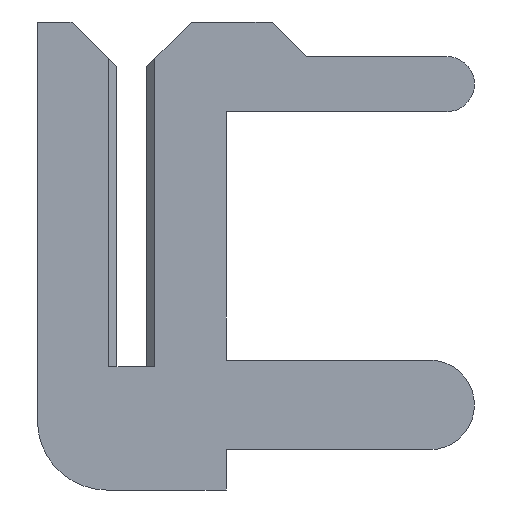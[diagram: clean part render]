
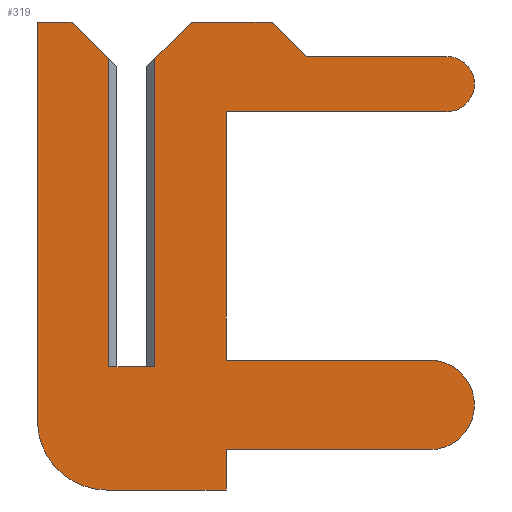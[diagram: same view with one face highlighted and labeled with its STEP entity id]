
A CAD part, left-side view. The second image highlights one B-rep face of the part: STEP entity #319.
In plain terms, the highlighted planar face has unit normal (-1, 0, 0).
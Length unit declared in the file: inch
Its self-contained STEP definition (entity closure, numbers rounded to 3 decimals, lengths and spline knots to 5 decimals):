
#2 = EDGE_CURVE ( 'NONE', #1011, #644, #802, .T. ) ;
#6 = AXIS2_PLACEMENT_3D ( 'NONE', #344, #510, #598 ) ;
#14 = LINE ( 'NONE', #711, #265 ) ;
#28 = EDGE_CURVE ( 'NONE', #370, #630, #1058, .T. ) ;
#31 = CIRCLE ( 'NONE', #512, 0.0195 ) ;
#42 = DIRECTION ( 'NONE',  ( 0., -1., 0. ) ) ;
#43 = EDGE_CURVE ( 'NONE', #541, #501, #550, .T. ) ;
#44 = CIRCLE ( 'NONE', #608, 0.03 ) ;
#46 = CARTESIAN_POINT ( 'NONE',  ( -0.01, -0.0065, 0.1305 ) ) ;
#52 = CARTESIAN_POINT ( 'NONE',  ( -0.01, 0.01, -0.0235 ) ) ;
#53 = CARTESIAN_POINT ( 'NONE',  ( -0.01, -0.1295, -0.0165 ) ) ;
#59 = EDGE_CURVE ( 'NONE', #644, #306, #841, .T. ) ;
#63 = PLANE ( 'NONE',  #1045 ) ;
#70 = CARTESIAN_POINT ( 'NONE',  ( -0.01, 0.011, -0.0235 ) ) ;
#73 = CARTESIAN_POINT ( 'NONE',  ( -0.01, -0.041, -0.036 ) ) ;
#79 = VERTEX_POINT ( 'NONE', #434 ) ;
#94 = CARTESIAN_POINT ( 'NONE',  ( -0.01, -0.137, 0.111 ) ) ;
#103 = LINE ( 'NONE', #46, #860 ) ;
#114 = CARTESIAN_POINT ( 'NONE',  ( -0.01, 0.041, 0.15 ) ) ;
#121 = ORIENTED_EDGE ( 'NONE', *, *, #570, .F. ) ;
#141 = DIRECTION ( 'NONE',  ( 0., 1., 0. ) ) ;
#142 = LINE ( 'NONE', #276, #324 ) ;
#153 = EDGE_CURVE ( 'NONE', #421, #204, #31, .T. ) ;
#160 = VECTOR ( 'NONE', #927, 39.37008 ) ;
#168 = EDGE_CURVE ( 'NONE', #865, #421, #820, .T. ) ;
#169 = LINE ( 'NONE', #288, #903 ) ;
#170 = EDGE_CURVE ( 'NONE', #611, #1011, #103, .T. ) ;
#179 = CARTESIAN_POINT ( 'NONE',  ( -0.01, 0.041, -0.0235 ) ) ;
#183 = LINE ( 'NONE', #674, #354 ) ;
#184 = LINE ( 'NONE', #73, #892 ) ;
#193 = DIRECTION ( 'NONE',  ( 0., 0., -1. ) ) ;
#204 = VERTEX_POINT ( 'NONE', #362 ) ;
#208 = DIRECTION ( 'NONE',  ( 0., 1., 0. ) ) ;
#217 = VECTOR ( 'NONE', #516, 39.37008 ) ;
#220 = ORIENTED_EDGE ( 'NONE', *, *, #698, .F. ) ;
#224 = CARTESIAN_POINT ( 'NONE',  ( -0.01, -0.01, 0. ) ) ;
#225 = DIRECTION ( 'NONE',  ( 0., 1., 0. ) ) ;
#247 = VERTEX_POINT ( 'NONE', #224 ) ;
#251 = EDGE_CURVE ( 'NONE', #501, #79, #14, .T. ) ;
#260 = ORIENTED_EDGE ( 'NONE', *, *, #59, .F. ) ;
#265 = VECTOR ( 'NONE', #525, 39.37008 ) ;
#273 = ORIENTED_EDGE ( 'NONE', *, *, #348, .F. ) ;
#276 = CARTESIAN_POINT ( 'NONE',  ( -0.01, -0.137, 0.135 ) ) ;
#277 = CARTESIAN_POINT ( 'NONE',  ( -0.01, -0.076, 0.135 ) ) ;
#282 = FACE_OUTER_BOUND ( 'NONE', #766, .T. ) ;
#288 = CARTESIAN_POINT ( 'NONE',  ( -0.01, -0.041, 0.111 ) ) ;
#294 = ORIENTED_EDGE ( 'NONE', *, *, #922, .T. ) ;
#296 = DIRECTION ( 'NONE',  ( 0., -0.707, 0.707 ) ) ;
#300 = ORIENTED_EDGE ( 'NONE', *, *, #792, .F. ) ;
#304 = CARTESIAN_POINT ( 'NONE',  ( -0.01, 0.01, 0.134 ) ) ;
#306 = VERTEX_POINT ( 'NONE', #796 ) ;
#319 = ADVANCED_FACE ( 'NONE', ( #282 ), #63, .T. ) ;
#324 = VECTOR ( 'NONE', #42, 39.37008 ) ;
#339 = CARTESIAN_POINT ( 'NONE',  ( -0.01, 0.011, -0.0235 ) ) ;
#342 = VERTEX_POINT ( 'NONE', #479 ) ;
#344 = CARTESIAN_POINT ( 'NONE',  ( -0.01, -0.137, 0.123 ) ) ;
#348 = EDGE_CURVE ( 'NONE', #204, #370, #184, .T. ) ;
#354 = VECTOR ( 'NONE', #594, 39.37008 ) ;
#356 = VECTOR ( 'NONE', #193, 39.37008 ) ;
#358 = DIRECTION ( 'NONE',  ( 0., -1., 0. ) ) ;
#362 = CARTESIAN_POINT ( 'NONE',  ( -0.01, -0.1295, -0.036 ) ) ;
#369 = VECTOR ( 'NONE', #720, 39.37008 ) ;
#370 = VERTEX_POINT ( 'NONE', #475 ) ;
#389 = ORIENTED_EDGE ( 'NONE', *, *, #476, .F. ) ;
#402 = EDGE_CURVE ( 'NONE', #611, #247, #590, .T. ) ;
#407 = CIRCLE ( 'NONE', #6, 0.012 ) ;
#408 = ORIENTED_EDGE ( 'NONE', *, *, #736, .F. ) ;
#414 = ORIENTED_EDGE ( 'NONE', *, *, #251, .F. ) ;
#418 = LINE ( 'NONE', #52, #561 ) ;
#421 = VERTEX_POINT ( 'NONE', #551 ) ;
#425 = CARTESIAN_POINT ( 'NONE',  ( -0.01, -0.137, 0.135 ) ) ;
#427 = ORIENTED_EDGE ( 'NONE', *, *, #170, .F. ) ;
#434 = CARTESIAN_POINT ( 'NONE',  ( -0.01, 0.026, 0.15 ) ) ;
#435 = CARTESIAN_POINT ( 'NONE',  ( -0.01, -0.041, 0.003 ) ) ;
#439 = DIRECTION ( 'NONE',  ( 0., -1., 0. ) ) ;
#445 = CARTESIAN_POINT ( 'NONE',  ( -0.01, -0.1295, 0.003 ) ) ;
#447 = CARTESIAN_POINT ( 'NONE',  ( -0.01, -0.041, 0.111 ) ) ;
#475 = CARTESIAN_POINT ( 'NONE',  ( -0.01, -0.041, -0.036 ) ) ;
#476 = EDGE_CURVE ( 'NONE', #79, #995, #520, .T. ) ;
#479 = CARTESIAN_POINT ( 'NONE',  ( -0.01, 0.01, 0. ) ) ;
#501 = VERTEX_POINT ( 'NONE', #985 ) ;
#504 = CARTESIAN_POINT ( 'NONE',  ( -0.01, 0.0065, 0. ) ) ;
#510 = DIRECTION ( 'NONE',  ( 1., 0., 0. ) ) ;
#512 = AXIS2_PLACEMENT_3D ( 'NONE', #53, #951, #784 ) ;
#516 = DIRECTION ( 'NONE',  ( 0., 0., 1. ) ) ;
#520 = LINE ( 'NONE', #902, #734 ) ;
#525 = DIRECTION ( 'NONE',  ( 0., -1., 0. ) ) ;
#541 = VERTEX_POINT ( 'NONE', #179 ) ;
#549 = VECTOR ( 'NONE', #439, 39.37008 ) ;
#550 = LINE ( 'NONE', #114, #217 ) ;
#551 = CARTESIAN_POINT ( 'NONE',  ( -0.01, -0.1295, 0.003 ) ) ;
#561 = VECTOR ( 'NONE', #609, 39.37008 ) ;
#570 = EDGE_CURVE ( 'NONE', #931, #541, #44, .T. ) ;
#571 = VERTEX_POINT ( 'NONE', #94 ) ;
#589 = LINE ( 'NONE', #504, #549 ) ;
#590 = LINE ( 'NONE', #960, #369 ) ;
#594 = DIRECTION ( 'NONE',  ( 0., 0., -1. ) ) ;
#598 = DIRECTION ( 'NONE',  ( 0., 0., 1. ) ) ;
#605 = ORIENTED_EDGE ( 'NONE', *, *, #168, .F. ) ;
#608 = AXIS2_PLACEMENT_3D ( 'NONE', #339, #999, #916 ) ;
#609 = DIRECTION ( 'NONE',  ( 0., 0., 1. ) ) ;
#611 = VERTEX_POINT ( 'NONE', #759 ) ;
#615 = ORIENTED_EDGE ( 'NONE', *, *, #402, .T. ) ;
#623 = ORIENTED_EDGE ( 'NONE', *, *, #153, .F. ) ;
#630 = VERTEX_POINT ( 'NONE', #755 ) ;
#632 = DIRECTION ( 'NONE',  ( -1., 0., 0. ) ) ;
#640 = DIRECTION ( 'NONE',  ( 0., 0., 1. ) ) ;
#644 = VERTEX_POINT ( 'NONE', #678 ) ;
#661 = VERTEX_POINT ( 'NONE', #425 ) ;
#674 = CARTESIAN_POINT ( 'NONE',  ( -0.01, -0.041, 0.003 ) ) ;
#678 = CARTESIAN_POINT ( 'NONE',  ( -0.01, -0.061, 0.15 ) ) ;
#688 = ORIENTED_EDGE ( 'NONE', *, *, #43, .F. ) ;
#690 = CARTESIAN_POINT ( 'NONE',  ( -0.01, 0.011, -0.0535 ) ) ;
#692 = CARTESIAN_POINT ( 'NONE',  ( -0.01, 0.011, -0.0535 ) ) ;
#698 = EDGE_CURVE ( 'NONE', #809, #865, #183, .T. ) ;
#711 = CARTESIAN_POINT ( 'NONE',  ( -0.01, 0.026, 0.15 ) ) ;
#720 = DIRECTION ( 'NONE',  ( 0., 0., -1. ) ) ;
#732 = DIRECTION ( 'NONE',  ( 0., -0.707, -0.707 ) ) ;
#734 = VECTOR ( 'NONE', #732, 39.37008 ) ;
#736 = EDGE_CURVE ( 'NONE', #661, #571, #407, .T. ) ;
#755 = CARTESIAN_POINT ( 'NONE',  ( -0.01, -0.041, -0.0535 ) ) ;
#759 = CARTESIAN_POINT ( 'NONE',  ( -0.01, -0.01, 0.134 ) ) ;
#760 = VECTOR ( 'NONE', #358, 39.37008 ) ;
#766 = EDGE_LOOP ( 'NONE', ( #427, #615, #300, #294, #389, #414, #688, #121, #978, #972, #273, #623, #605, #220, #834, #408, #1051, #260, #981 ) ) ;
#772 = CARTESIAN_POINT ( 'NONE',  ( -0.01, -0.041, -0.0535 ) ) ;
#784 = DIRECTION ( 'NONE',  ( 0., 0., 1. ) ) ;
#786 = DIRECTION ( 'NONE',  ( 0., -1., 0. ) ) ;
#789 = VECTOR ( 'NONE', #786, 39.37008 ) ;
#792 = EDGE_CURVE ( 'NONE', #342, #247, #589, .T. ) ;
#796 = CARTESIAN_POINT ( 'NONE',  ( -0.01, -0.076, 0.135 ) ) ;
#802 = LINE ( 'NONE', #1008, #760 ) ;
#809 = VERTEX_POINT ( 'NONE', #447 ) ;
#817 = EDGE_CURVE ( 'NONE', #630, #931, #914, .T. ) ;
#820 = LINE ( 'NONE', #445, #789 ) ;
#834 = ORIENTED_EDGE ( 'NONE', *, *, #974, .F. ) ;
#841 = LINE ( 'NONE', #277, #160 ) ;
#860 = VECTOR ( 'NONE', #296, 39.37008 ) ;
#865 = VERTEX_POINT ( 'NONE', #435 ) ;
#887 = EDGE_CURVE ( 'NONE', #306, #661, #142, .T. ) ;
#892 = VECTOR ( 'NONE', #141, 39.37008 ) ;
#902 = CARTESIAN_POINT ( 'NONE',  ( -0.01, 0.0065, 0.1305 ) ) ;
#903 = VECTOR ( 'NONE', #225, 39.37008 ) ;
#914 = LINE ( 'NONE', #690, #977 ) ;
#916 = DIRECTION ( 'NONE',  ( 0., 0., 1. ) ) ;
#922 = EDGE_CURVE ( 'NONE', #342, #995, #418, .T. ) ;
#927 = DIRECTION ( 'NONE',  ( 0., -0.707, -0.707 ) ) ;
#931 = VERTEX_POINT ( 'NONE', #692 ) ;
#951 = DIRECTION ( 'NONE',  ( 1., 0., 0. ) ) ;
#957 = CARTESIAN_POINT ( 'NONE',  ( -0.01, -0.026, 0.15 ) ) ;
#960 = CARTESIAN_POINT ( 'NONE',  ( -0.01, -0.01, 0.15 ) ) ;
#972 = ORIENTED_EDGE ( 'NONE', *, *, #28, .F. ) ;
#974 = EDGE_CURVE ( 'NONE', #571, #809, #169, .T. ) ;
#977 = VECTOR ( 'NONE', #208, 39.37008 ) ;
#978 = ORIENTED_EDGE ( 'NONE', *, *, #817, .F. ) ;
#981 = ORIENTED_EDGE ( 'NONE', *, *, #2, .F. ) ;
#985 = CARTESIAN_POINT ( 'NONE',  ( -0.01, 0.041, 0.15 ) ) ;
#995 = VERTEX_POINT ( 'NONE', #304 ) ;
#999 = DIRECTION ( 'NONE',  ( 1., 0., 0. ) ) ;
#1008 = CARTESIAN_POINT ( 'NONE',  ( -0.01, -0.026, 0.15 ) ) ;
#1011 = VERTEX_POINT ( 'NONE', #957 ) ;
#1045 = AXIS2_PLACEMENT_3D ( 'NONE', #70, #632, #640 ) ;
#1051 = ORIENTED_EDGE ( 'NONE', *, *, #887, .F. ) ;
#1058 = LINE ( 'NONE', #772, #356 ) ;
